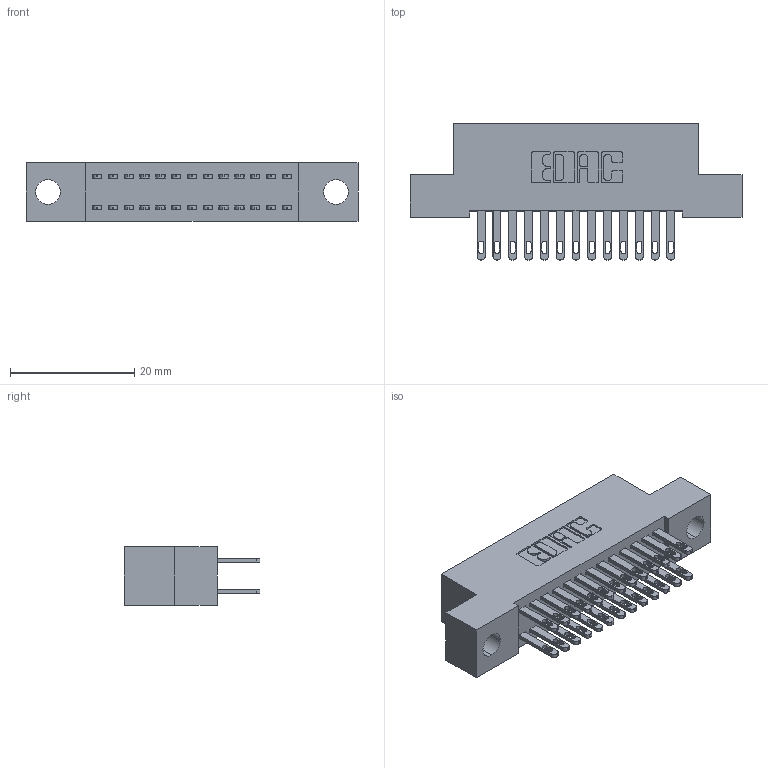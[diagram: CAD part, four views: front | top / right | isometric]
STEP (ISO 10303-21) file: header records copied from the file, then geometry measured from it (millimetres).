
FILE_DESCRIPTION (( 'STEP AP203' ), '1' );
FILE_NAME ('892-026-500-204.STEP', '2020-09-21T14:41:09', ( '' ), ( '' ), 'SwSTEP 2.0', 'SolidWorks 2020', '' );
FILE_SCHEMA (( 'CONFIG_CONTROL_DESIGN' ));
Length unit declared in the file: inch
Products named in the file (3): 345-292-001_345-293-100; 892-026-500-204; 842 Part_.156 TH
Assembly tree (27 placements, depth 2):
  892-026-500-204
    842 Part_.156 TH
    345-292-001_345-293-100  x26
Bounding box: 53.34 x 21.85 x 9.4 mm (x, y, z)
Volume: 4647.8 mm3; surface area: 6923.9 mm2
Topology: 27 solids, 27 shells, 1358 faces, 4121 edges, 2746 vertices
Faces by surface type: plane 846, cylinder 512
Entity records: 11915 total; most frequent: CARTESIAN_POINT 2006, ORIENTED_EDGE 1942, DIRECTION 1767, EDGE_CURVE 971, LINE 839, VECTOR 839, VERTEX_POINT 646, AXIS2_PLACEMENT_3D 464
